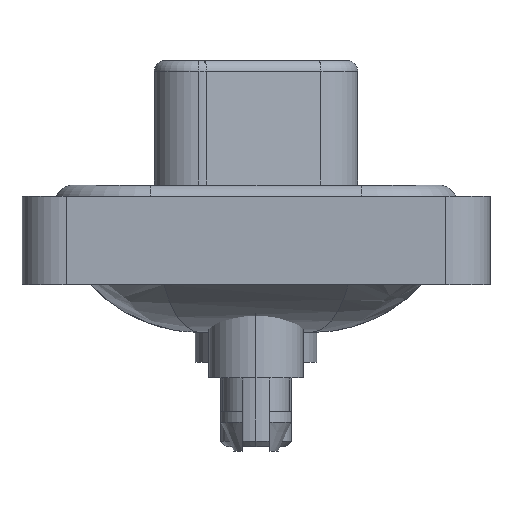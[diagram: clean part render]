
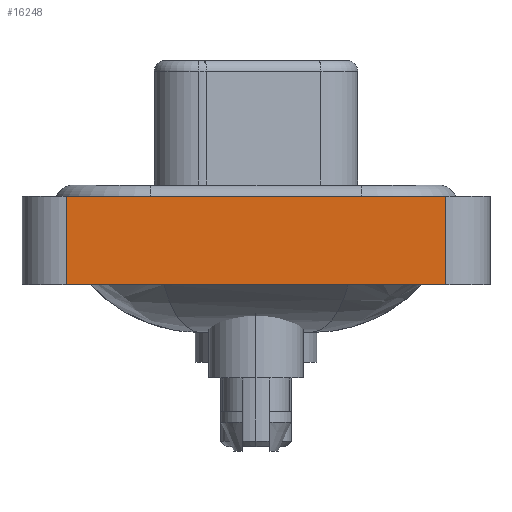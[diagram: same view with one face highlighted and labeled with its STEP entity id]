
A CAD part, left-side view. The second image highlights one B-rep face of the part: STEP entity #16248.
In plain terms, the highlighted planar face has unit normal (-1, 0, 0).
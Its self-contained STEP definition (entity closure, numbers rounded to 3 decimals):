
#360 = VECTOR ( 'NONE', #17938, 1000. ) ;
#1157 = DIRECTION ( 'NONE',  ( -1., 0., 0. ) ) ;
#1164 = VECTOR ( 'NONE', #7862, 1000. ) ;
#3497 = AXIS2_PLACEMENT_3D ( 'NONE', #15918, #1157, #3925 ) ;
#3542 = EDGE_CURVE ( 'NONE', #9738, #6993, #3610, .T. ) ;
#3610 = LINE ( 'NONE', #15331, #1164 ) ;
#3873 = EDGE_LOOP ( 'NONE', ( #6256, #11032, #14158, #8979 ) ) ;
#3925 = DIRECTION ( 'NONE',  ( 0., 0., 1. ) ) ;
#4257 = LINE ( 'NONE', #8629, #7292 ) ;
#5271 = DIRECTION ( 'NONE',  ( 0., 0., 1. ) ) ;
#5519 = CARTESIAN_POINT ( 'NONE',  ( -7.35, 8.55, -3.6 ) ) ;
#5534 = PLANE ( 'NONE',  #3497 ) ;
#5957 = DIRECTION ( 'NONE',  ( 0., -1., 0. ) ) ;
#6256 = ORIENTED_EDGE ( 'NONE', *, *, #3542, .T. ) ;
#6353 = CARTESIAN_POINT ( 'NONE',  ( -7.35, 8.55, 0.4 ) ) ;
#6962 = CARTESIAN_POINT ( 'NONE',  ( -7.35, 8.55, -3.6 ) ) ;
#6993 = VERTEX_POINT ( 'NONE', #10886 ) ;
#7292 = VECTOR ( 'NONE', #5957, 1000. ) ;
#7862 = DIRECTION ( 'NONE',  ( 0., 0., 1. ) ) ;
#8629 = CARTESIAN_POINT ( 'NONE',  ( -7.35, -8.55, -3.6 ) ) ;
#8635 = EDGE_CURVE ( 'NONE', #9106, #13284, #9550, .T. ) ;
#8709 = VECTOR ( 'NONE', #5271, 1000. ) ;
#8979 = ORIENTED_EDGE ( 'NONE', *, *, #10962, .T. ) ;
#9065 = LINE ( 'NONE', #12119, #360 ) ;
#9106 = VERTEX_POINT ( 'NONE', #5519 ) ;
#9550 = LINE ( 'NONE', #6962, #8709 ) ;
#9738 = VERTEX_POINT ( 'NONE', #13845 ) ;
#10886 = CARTESIAN_POINT ( 'NONE',  ( -7.35, -8.55, 0.4 ) ) ;
#10962 = EDGE_CURVE ( 'NONE', #9106, #9738, #4257, .T. ) ;
#11032 = ORIENTED_EDGE ( 'NONE', *, *, #11552, .F. ) ;
#11552 = EDGE_CURVE ( 'NONE', #13284, #6993, #9065, .T. ) ;
#12119 = CARTESIAN_POINT ( 'NONE',  ( -7.35, -8.55, 0.4 ) ) ;
#13284 = VERTEX_POINT ( 'NONE', #6353 ) ;
#13845 = CARTESIAN_POINT ( 'NONE',  ( -7.35, -8.55, -3.6 ) ) ;
#14158 = ORIENTED_EDGE ( 'NONE', *, *, #8635, .F. ) ;
#15331 = CARTESIAN_POINT ( 'NONE',  ( -7.35, -8.55, -3.6 ) ) ;
#15918 = CARTESIAN_POINT ( 'NONE',  ( -7.35, -8.55, -3.6 ) ) ;
#16248 = ADVANCED_FACE ( 'NONE', ( #17340 ), #5534, .T. ) ;
#17340 = FACE_OUTER_BOUND ( 'NONE', #3873, .T. ) ;
#17938 = DIRECTION ( 'NONE',  ( 0., -1., 0. ) ) ;
